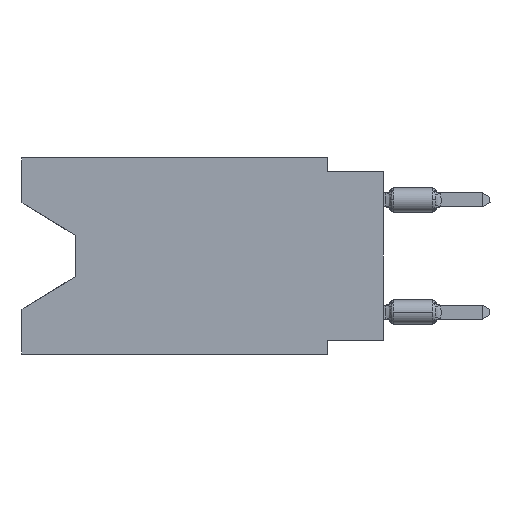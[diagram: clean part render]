
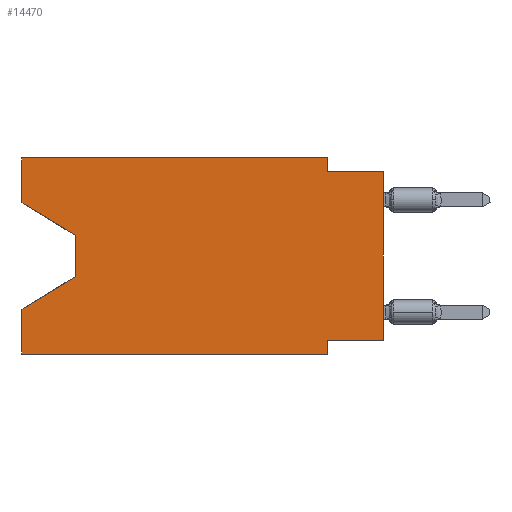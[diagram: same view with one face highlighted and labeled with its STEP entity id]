
A CAD part, left-side view. The second image highlights one B-rep face of the part: STEP entity #14470.
In plain terms, the highlighted planar face has unit normal (-1, 0, 0).
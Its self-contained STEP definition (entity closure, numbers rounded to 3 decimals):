
#126 = VECTOR ( 'NONE', #42423, 1000. ) ;
#1211 = VECTOR ( 'NONE', #10368, 1000. ) ;
#1998 = DIRECTION ( 'NONE',  ( 0., -1., 0. ) ) ;
#2081 = LINE ( 'NONE', #32265, #3228 ) ;
#2206 = CARTESIAN_POINT ( 'NONE',  ( 0., 2.54, -8.89 ) ) ;
#2302 = ORIENTED_EDGE ( 'NONE', *, *, #8739, .F. ) ;
#3048 = LINE ( 'NONE', #3319, #27288 ) ;
#3228 = VECTOR ( 'NONE', #18982, 1000. ) ;
#3319 = CARTESIAN_POINT ( 'NONE',  ( 0., 16.383, 0. ) ) ;
#4087 = ORIENTED_EDGE ( 'NONE', *, *, #10635, .F. ) ;
#4958 = EDGE_CURVE ( 'NONE', #47595, #17962, #2081, .T. ) ;
#5889 = LINE ( 'NONE', #14742, #9433 ) ;
#6398 = VECTOR ( 'NONE', #32493, 1000. ) ;
#6966 = EDGE_CURVE ( 'NONE', #46802, #36860, #5889, .T. ) ;
#7779 = DIRECTION ( 'NONE',  ( 0., -0.855, -0.519 ) ) ;
#8495 = CARTESIAN_POINT ( 'NONE',  ( 0., 0., -8.255 ) ) ;
#8739 = EDGE_CURVE ( 'NONE', #31049, #14091, #3048, .T. ) ;
#9247 = LINE ( 'NONE', #51031, #26805 ) ;
#9433 = VECTOR ( 'NONE', #1998, 1000. ) ;
#9489 = ORIENTED_EDGE ( 'NONE', *, *, #14820, .T. ) ;
#9627 = ORIENTED_EDGE ( 'NONE', *, *, #53908, .T. ) ;
#9839 = ORIENTED_EDGE ( 'NONE', *, *, #4958, .T. ) ;
#10368 = DIRECTION ( 'NONE',  ( 0., 0.855, -0.519 ) ) ;
#10635 = EDGE_CURVE ( 'NONE', #47261, #31644, #18570, .T. ) ;
#11073 = ORIENTED_EDGE ( 'NONE', *, *, #6966, .T. ) ;
#11851 = EDGE_CURVE ( 'NONE', #14091, #15801, #25883, .T. ) ;
#13543 = CARTESIAN_POINT ( 'NONE',  ( 0., 2.54, -0.635 ) ) ;
#13669 = CARTESIAN_POINT ( 'NONE',  ( 0., 0., -0.635 ) ) ;
#14091 = VERTEX_POINT ( 'NONE', #29022 ) ;
#14128 = ORIENTED_EDGE ( 'NONE', *, *, #46880, .F. ) ;
#14470 = ADVANCED_FACE ( 'NONE', ( #18719 ), #31454, .F. ) ;
#14742 = CARTESIAN_POINT ( 'NONE',  ( 0., 16.383, -8.89 ) ) ;
#14820 = EDGE_CURVE ( 'NONE', #17962, #25814, #27803, .T. ) ;
#15529 = EDGE_LOOP ( 'NONE', ( #51685, #9839, #9489, #28138, #11073, #41413, #14128, #9627, #4087, #32679, #36955, #2302 ) ) ;
#15801 = VERTEX_POINT ( 'NONE', #36726 ) ;
#17433 = CARTESIAN_POINT ( 'NONE',  ( 0., 16.383, -2.038 ) ) ;
#17569 = CARTESIAN_POINT ( 'NONE',  ( 0., 13.97, -5.385 ) ) ;
#17832 = DIRECTION ( 'NONE',  ( 0., -1., 0. ) ) ;
#17962 = VERTEX_POINT ( 'NONE', #17569 ) ;
#18454 = LINE ( 'NONE', #23443, #36796 ) ;
#18570 = LINE ( 'NONE', #36559, #49521 ) ;
#18719 = FACE_OUTER_BOUND ( 'NONE', #15529, .T. ) ;
#18982 = DIRECTION ( 'NONE',  ( 0., 0., -1. ) ) ;
#21323 = VECTOR ( 'NONE', #17832, 1000. ) ;
#21812 = CARTESIAN_POINT ( 'NONE',  ( 0., 16.383, -8.89 ) ) ;
#22443 = EDGE_CURVE ( 'NONE', #54304, #36860, #26635, .T. ) ;
#23443 = CARTESIAN_POINT ( 'NONE',  ( 0., 0., -8.255 ) ) ;
#25299 = VERTEX_POINT ( 'NONE', #8495 ) ;
#25814 = VERTEX_POINT ( 'NONE', #54451 ) ;
#25883 = LINE ( 'NONE', #30577, #21323 ) ;
#26635 = LINE ( 'NONE', #43520, #126 ) ;
#26805 = VECTOR ( 'NONE', #29995, 1000. ) ;
#27288 = VECTOR ( 'NONE', #41244, 1000. ) ;
#27803 = LINE ( 'NONE', #39685, #1211 ) ;
#28138 = ORIENTED_EDGE ( 'NONE', *, *, #53012, .F. ) ;
#29022 = CARTESIAN_POINT ( 'NONE',  ( 0., 16.383, 0. ) ) ;
#29367 = LINE ( 'NONE', #17433, #44211 ) ;
#29438 = LINE ( 'NONE', #46034, #6398 ) ;
#29551 = VECTOR ( 'NONE', #36583, 1000. ) ;
#29995 = DIRECTION ( 'NONE',  ( 0., 0., 1. ) ) ;
#30577 = CARTESIAN_POINT ( 'NONE',  ( 0., 16.383, 0. ) ) ;
#31049 = VERTEX_POINT ( 'NONE', #33094 ) ;
#31182 = DIRECTION ( 'NONE',  ( 0., 0., -1. ) ) ;
#31454 = PLANE ( 'NONE',  #40981 ) ;
#31644 = VERTEX_POINT ( 'NONE', #13669 ) ;
#32265 = CARTESIAN_POINT ( 'NONE',  ( 0., 13.97, -3.505 ) ) ;
#32493 = DIRECTION ( 'NONE',  ( 0., 0., 1. ) ) ;
#32679 = ORIENTED_EDGE ( 'NONE', *, *, #33503, .F. ) ;
#32696 = CARTESIAN_POINT ( 'NONE',  ( 0., 2.54, 0. ) ) ;
#33094 = CARTESIAN_POINT ( 'NONE',  ( 0., 16.383, -2.038 ) ) ;
#33503 = EDGE_CURVE ( 'NONE', #15801, #47261, #49045, .T. ) ;
#36559 = CARTESIAN_POINT ( 'NONE',  ( 0., 0., -0.635 ) ) ;
#36583 = DIRECTION ( 'NONE',  ( 0., 0., -1. ) ) ;
#36726 = CARTESIAN_POINT ( 'NONE',  ( 0., 2.54, 0. ) ) ;
#36796 = VECTOR ( 'NONE', #40309, 1000. ) ;
#36860 = VERTEX_POINT ( 'NONE', #2206 ) ;
#36955 = ORIENTED_EDGE ( 'NONE', *, *, #11851, .F. ) ;
#39685 = CARTESIAN_POINT ( 'NONE',  ( 0., 13.97, -5.385 ) ) ;
#40023 = DIRECTION ( 'NONE',  ( 1., 0., 0. ) ) ;
#40309 = DIRECTION ( 'NONE',  ( 0., 1., 0. ) ) ;
#40981 = AXIS2_PLACEMENT_3D ( 'NONE', #44177, #40023, #31182 ) ;
#41244 = DIRECTION ( 'NONE',  ( 0., 0., 1. ) ) ;
#41413 = ORIENTED_EDGE ( 'NONE', *, *, #22443, .F. ) ;
#42423 = DIRECTION ( 'NONE',  ( 0., 0., -1. ) ) ;
#43520 = CARTESIAN_POINT ( 'NONE',  ( 0., 2.54, -8.89 ) ) ;
#44177 = CARTESIAN_POINT ( 'NONE',  ( 0., 16.383, 0. ) ) ;
#44211 = VECTOR ( 'NONE', #7779, 1000. ) ;
#44448 = CARTESIAN_POINT ( 'NONE',  ( 0., 13.97, -3.505 ) ) ;
#46034 = CARTESIAN_POINT ( 'NONE',  ( 0., 16.383, 0. ) ) ;
#46552 = CARTESIAN_POINT ( 'NONE',  ( 0., 2.54, -8.255 ) ) ;
#46802 = VERTEX_POINT ( 'NONE', #21812 ) ;
#46880 = EDGE_CURVE ( 'NONE', #25299, #54304, #18454, .T. ) ;
#47261 = VERTEX_POINT ( 'NONE', #13543 ) ;
#47595 = VERTEX_POINT ( 'NONE', #44448 ) ;
#48746 = DIRECTION ( 'NONE',  ( 0., -1., 0. ) ) ;
#49045 = LINE ( 'NONE', #32696, #29551 ) ;
#49521 = VECTOR ( 'NONE', #48746, 1000. ) ;
#51031 = CARTESIAN_POINT ( 'NONE',  ( 0., 0., 0. ) ) ;
#51685 = ORIENTED_EDGE ( 'NONE', *, *, #51794, .T. ) ;
#51794 = EDGE_CURVE ( 'NONE', #31049, #47595, #29367, .T. ) ;
#53012 = EDGE_CURVE ( 'NONE', #46802, #25814, #29438, .T. ) ;
#53908 = EDGE_CURVE ( 'NONE', #25299, #31644, #9247, .T. ) ;
#54304 = VERTEX_POINT ( 'NONE', #46552 ) ;
#54451 = CARTESIAN_POINT ( 'NONE',  ( 0., 16.383, -6.852 ) ) ;
